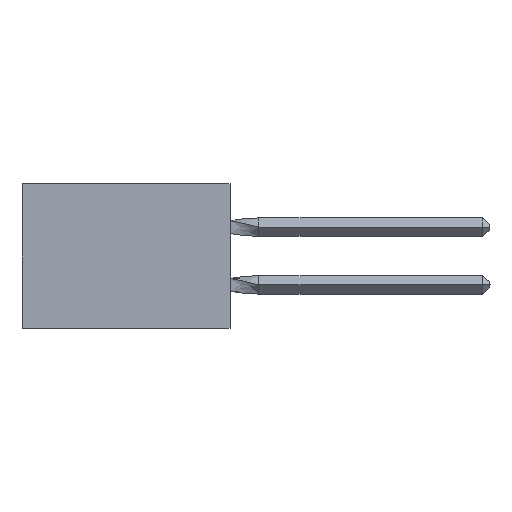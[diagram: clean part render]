
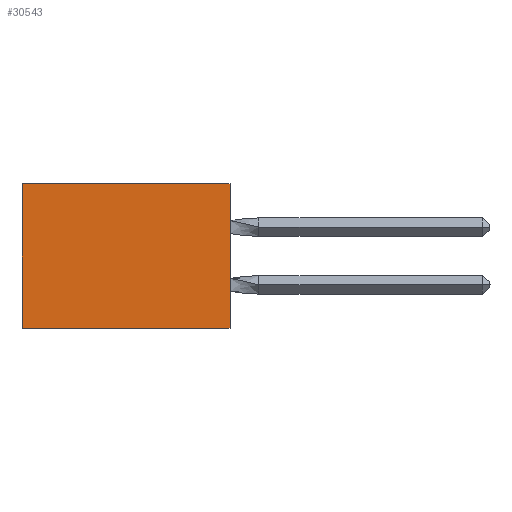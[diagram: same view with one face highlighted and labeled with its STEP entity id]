
A CAD part, left-side view. The second image highlights one B-rep face of the part: STEP entity #30543.
In plain terms, the highlighted planar face has unit normal (-1, 0, 0).
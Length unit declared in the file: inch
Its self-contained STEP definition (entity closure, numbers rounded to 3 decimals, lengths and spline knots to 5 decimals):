
#1209 = VERTEX_POINT ( 'NONE', #9065 ) ;
#2720 = DIRECTION ( 'NONE',  ( 0., 0., -1. ) ) ;
#2769 = DIRECTION ( 'NONE',  ( 1., 0., 0. ) ) ;
#2832 = ORIENTED_EDGE ( 'NONE', *, *, #25829, .T. ) ;
#4791 = ORIENTED_EDGE ( 'NONE', *, *, #6882, .F. ) ;
#5380 = AXIS2_PLACEMENT_3D ( 'NONE', #25926, #2769, #10626 ) ;
#6381 = VECTOR ( 'NONE', #6972, 39.37008 ) ;
#6882 = EDGE_CURVE ( 'NONE', #16777, #23252, #31099, .T. ) ;
#6972 = DIRECTION ( 'NONE',  ( 0., 0., -1. ) ) ;
#7932 = PLANE ( 'NONE',  #5380 ) ;
#7943 = DIRECTION ( 'NONE',  ( 0., 1., 0. ) ) ;
#9065 = CARTESIAN_POINT ( 'NONE',  ( 0.305, 0.72, -0.5 ) ) ;
#10626 = DIRECTION ( 'NONE',  ( 0., 0., -1. ) ) ;
#11487 = LINE ( 'NONE', #15826, #21356 ) ;
#14796 = CARTESIAN_POINT ( 'NONE',  ( 0.305, 0., -0.5 ) ) ;
#15826 = CARTESIAN_POINT ( 'NONE',  ( 0.305, 0.72, -0.5 ) ) ;
#15907 = EDGE_LOOP ( 'NONE', ( #23923, #30519, #4791, #2832 ) ) ;
#16697 = CARTESIAN_POINT ( 'NONE',  ( 0.305, 0., 0. ) ) ;
#16777 = VERTEX_POINT ( 'NONE', #16697 ) ;
#16781 = VECTOR ( 'NONE', #23969, 39.37008 ) ;
#16999 = FACE_OUTER_BOUND ( 'NONE', #15907, .T. ) ;
#17116 = EDGE_CURVE ( 'NONE', #23252, #1209, #28297, .T. ) ;
#18902 = CARTESIAN_POINT ( 'NONE',  ( 0.305, 0., -0.5 ) ) ;
#18918 = LINE ( 'NONE', #29264, #24288 ) ;
#21356 = VECTOR ( 'NONE', #2720, 39.37008 ) ;
#23252 = VERTEX_POINT ( 'NONE', #29222 ) ;
#23923 = ORIENTED_EDGE ( 'NONE', *, *, #27983, .T. ) ;
#23969 = DIRECTION ( 'NONE',  ( 0., 1., 0. ) ) ;
#24288 = VECTOR ( 'NONE', #7943, 39.37008 ) ;
#24303 = CARTESIAN_POINT ( 'NONE',  ( 0.305, 0.72, 0. ) ) ;
#24502 = VERTEX_POINT ( 'NONE', #24303 ) ;
#25829 = EDGE_CURVE ( 'NONE', #16777, #24502, #18918, .T. ) ;
#25926 = CARTESIAN_POINT ( 'NONE',  ( 0.305, 0., -0.5 ) ) ;
#27983 = EDGE_CURVE ( 'NONE', #24502, #1209, #11487, .T. ) ;
#28297 = LINE ( 'NONE', #18902, #16781 ) ;
#29222 = CARTESIAN_POINT ( 'NONE',  ( 0.305, 0., -0.5 ) ) ;
#29264 = CARTESIAN_POINT ( 'NONE',  ( 0.305, 0., 0. ) ) ;
#30519 = ORIENTED_EDGE ( 'NONE', *, *, #17116, .F. ) ;
#30543 = ADVANCED_FACE ( 'NONE', ( #16999 ), #7932, .F. ) ;
#31099 = LINE ( 'NONE', #14796, #6381 ) ;
